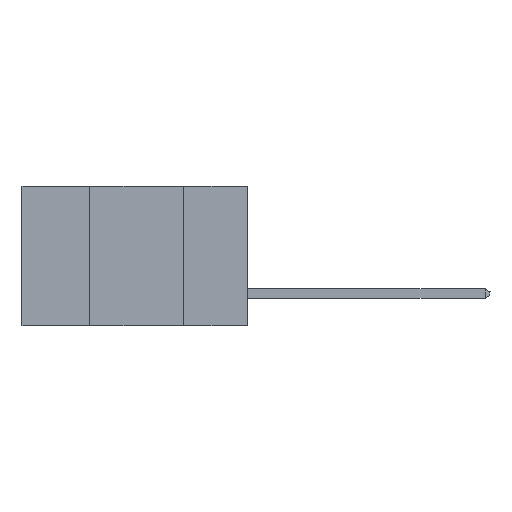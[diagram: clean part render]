
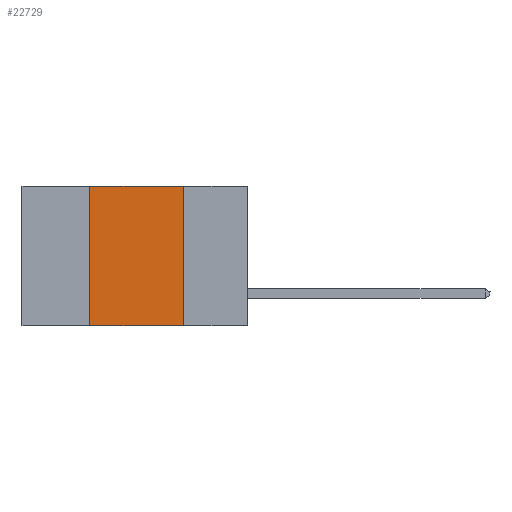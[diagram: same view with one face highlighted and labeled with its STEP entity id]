
A CAD part, left-side view. The second image highlights one B-rep face of the part: STEP entity #22729.
In plain terms, the highlighted planar face has unit normal (-1, 0, 0).
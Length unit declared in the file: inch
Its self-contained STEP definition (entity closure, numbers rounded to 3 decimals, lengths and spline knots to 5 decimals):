
#483 = VECTOR ( 'NONE', #2977, 39.37008 ) ;
#873 = CARTESIAN_POINT ( 'NONE',  ( 0., 0.42, -0.37 ) ) ;
#2061 = CARTESIAN_POINT ( 'NONE',  ( 0., 0.6, 0. ) ) ;
#2276 = VECTOR ( 'NONE', #10225, 39.37008 ) ;
#2381 = CARTESIAN_POINT ( 'NONE',  ( 0., 0.17, -0.37 ) ) ;
#2977 = DIRECTION ( 'NONE',  ( 0., -1., 0. ) ) ;
#3359 = CARTESIAN_POINT ( 'NONE',  ( 0., 0.6, 0. ) ) ;
#3758 = ORIENTED_EDGE ( 'NONE', *, *, #6795, .F. ) ;
#4045 = VECTOR ( 'NONE', #4251, 39.37008 ) ;
#4251 = DIRECTION ( 'NONE',  ( 0., 0., -1. ) ) ;
#4489 = ORIENTED_EDGE ( 'NONE', *, *, #10483, .F. ) ;
#5730 = PLANE ( 'NONE',  #19952 ) ;
#5806 = DIRECTION ( 'NONE',  ( 0., 0., -1. ) ) ;
#6038 = LINE ( 'NONE', #3359, #483 ) ;
#6795 = EDGE_CURVE ( 'NONE', #12820, #22548, #6038, .T. ) ;
#6921 = FACE_OUTER_BOUND ( 'NONE', #14741, .T. ) ;
#7575 = ORIENTED_EDGE ( 'NONE', *, *, #22833, .F. ) ;
#8405 = CARTESIAN_POINT ( 'NONE',  ( 0., 0.6, -0.37 ) ) ;
#10225 = DIRECTION ( 'NONE',  ( 0., -1., 0. ) ) ;
#10483 = EDGE_CURVE ( 'NONE', #22723, #12820, #16318, .T. ) ;
#12033 = DIRECTION ( 'NONE',  ( 0., 0., 1. ) ) ;
#12820 = VERTEX_POINT ( 'NONE', #20255 ) ;
#13636 = ORIENTED_EDGE ( 'NONE', *, *, #15393, .T. ) ;
#14741 = EDGE_LOOP ( 'NONE', ( #7575, #3758, #4489, #13636 ) ) ;
#15393 = EDGE_CURVE ( 'NONE', #22723, #15455, #16894, .T. ) ;
#15455 = VERTEX_POINT ( 'NONE', #17588 ) ;
#16318 = LINE ( 'NONE', #873, #19850 ) ;
#16724 = DIRECTION ( 'NONE',  ( 1., 0., 0. ) ) ;
#16894 = LINE ( 'NONE', #8405, #2276 ) ;
#17588 = CARTESIAN_POINT ( 'NONE',  ( 0., 0.17, -0.37 ) ) ;
#17952 = CARTESIAN_POINT ( 'NONE',  ( 0., 0.17, 0. ) ) ;
#18543 = LINE ( 'NONE', #2381, #4045 ) ;
#19850 = VECTOR ( 'NONE', #12033, 39.37008 ) ;
#19952 = AXIS2_PLACEMENT_3D ( 'NONE', #2061, #16724, #5806 ) ;
#20255 = CARTESIAN_POINT ( 'NONE',  ( 0., 0.42, 0. ) ) ;
#21894 = CARTESIAN_POINT ( 'NONE',  ( 0., 0.42, -0.37 ) ) ;
#22548 = VERTEX_POINT ( 'NONE', #17952 ) ;
#22723 = VERTEX_POINT ( 'NONE', #21894 ) ;
#22729 = ADVANCED_FACE ( 'NONE', ( #6921 ), #5730, .F. ) ;
#22833 = EDGE_CURVE ( 'NONE', #22548, #15455, #18543, .T. ) ;
